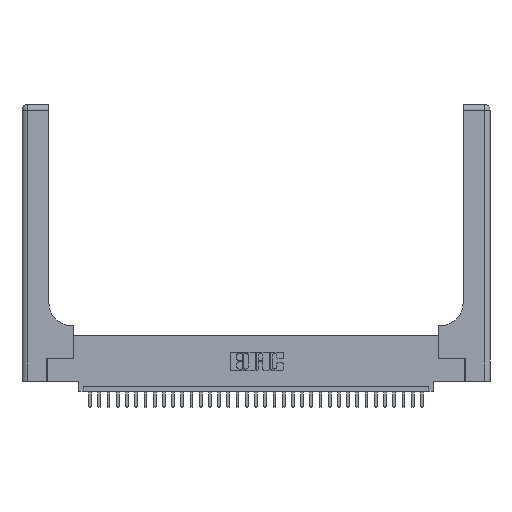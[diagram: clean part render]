
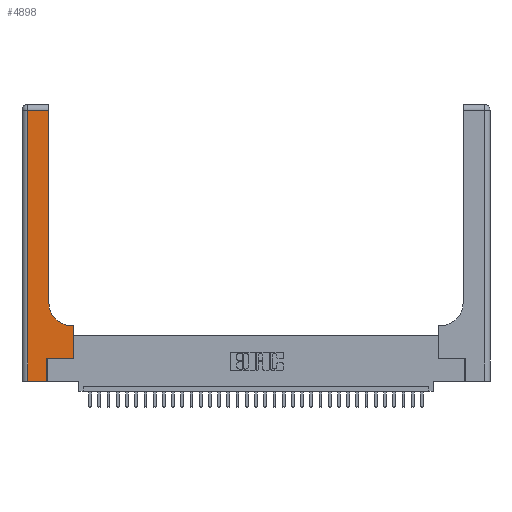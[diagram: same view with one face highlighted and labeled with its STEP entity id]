
A CAD part, top view. The second image highlights one B-rep face of the part: STEP entity #4898.
In plain terms, the highlighted planar face has unit normal (0, 0, 1).
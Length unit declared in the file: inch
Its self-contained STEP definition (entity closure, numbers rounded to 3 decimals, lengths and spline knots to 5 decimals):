
#101 = VERTEX_POINT ( 'NONE', #15010 ) ;
#914 = VERTEX_POINT ( 'NONE', #10750 ) ;
#1410 = CARTESIAN_POINT ( 'NONE',  ( 0.06, 3., 0.37 ) ) ;
#1652 = CARTESIAN_POINT ( 'NONE',  ( 0.5585, 0.6, 0.37 ) ) ;
#3017 = DIRECTION ( 'NONE',  ( 0., 1., 0. ) ) ;
#3112 = EDGE_CURVE ( 'NONE', #20551, #27296, #12421, .T. ) ;
#3585 = CARTESIAN_POINT ( 'NONE',  ( 0., 2.94, 0.37 ) ) ;
#4898 = ADVANCED_FACE ( 'NONE', ( #30278 ), #31726, .F. ) ;
#5495 = DIRECTION ( 'NONE',  ( 0., 0., -1. ) ) ;
#5794 = LINE ( 'NONE', #6633, #22554 ) ;
#5847 = ORIENTED_EDGE ( 'NONE', *, *, #11827, .T. ) ;
#5917 = VERTEX_POINT ( 'NONE', #32059 ) ;
#6014 = CIRCLE ( 'NONE', #30417, 0.25 ) ;
#6218 = DIRECTION ( 'NONE',  ( 0., -1., 0. ) ) ;
#6274 = DIRECTION ( 'NONE',  ( 0., 1., 0. ) ) ;
#6325 = ORIENTED_EDGE ( 'NONE', *, *, #32760, .T. ) ;
#6549 = VECTOR ( 'NONE', #22015, 39.37008 ) ;
#6633 = CARTESIAN_POINT ( 'NONE',  ( 0.5585, 0.25, 0.37 ) ) ;
#7405 = LINE ( 'NONE', #21415, #28686 ) ;
#8240 = CARTESIAN_POINT ( 'NONE',  ( 0., 3., 0.37 ) ) ;
#8337 = LINE ( 'NONE', #1410, #32090 ) ;
#8367 = DIRECTION ( 'NONE',  ( 1., 0., 0. ) ) ;
#8382 = EDGE_CURVE ( 'NONE', #914, #101, #29409, .T. ) ;
#8520 = CARTESIAN_POINT ( 'NONE',  ( 0.269, 0., 0.37 ) ) ;
#8709 = ORIENTED_EDGE ( 'NONE', *, *, #16047, .T. ) ;
#9122 = ORIENTED_EDGE ( 'NONE', *, *, #3112, .T. ) ;
#9137 = VERTEX_POINT ( 'NONE', #15491 ) ;
#9148 = DIRECTION ( 'NONE',  ( 0., 0., -1. ) ) ;
#9297 = ORIENTED_EDGE ( 'NONE', *, *, #15444, .T. ) ;
#9334 = VECTOR ( 'NONE', #6274, 39.37008 ) ;
#9368 = DIRECTION ( 'NONE',  ( 0., 1., 0. ) ) ;
#10034 = AXIS2_PLACEMENT_3D ( 'NONE', #8240, #5495, #16240 ) ;
#10750 = CARTESIAN_POINT ( 'NONE',  ( 0.269, 0.25, 0.37 ) ) ;
#11162 = DIRECTION ( 'NONE',  ( 1., 0., 0. ) ) ;
#11827 = EDGE_CURVE ( 'NONE', #5917, #28578, #15257, .T. ) ;
#12421 = LINE ( 'NONE', #21378, #31283 ) ;
#12800 = CARTESIAN_POINT ( 'NONE',  ( 0.06, 0., 0.37 ) ) ;
#13946 = CARTESIAN_POINT ( 'NONE',  ( 0.2915, 3., 0.37 ) ) ;
#14524 = EDGE_CURVE ( 'NONE', #28578, #20551, #8337, .T. ) ;
#14715 = EDGE_LOOP ( 'NONE', ( #21455, #5847, #18356, #9122, #15242, #21396, #9297, #8709, #6325 ) ) ;
#15010 = CARTESIAN_POINT ( 'NONE',  ( 0.5585, 0.25, 0.37 ) ) ;
#15242 = ORIENTED_EDGE ( 'NONE', *, *, #26597, .T. ) ;
#15257 = LINE ( 'NONE', #3585, #28356 ) ;
#15444 = EDGE_CURVE ( 'NONE', #101, #21053, #5794, .T. ) ;
#15491 = CARTESIAN_POINT ( 'NONE',  ( 0.5415, 0.6, 0.37 ) ) ;
#16047 = EDGE_CURVE ( 'NONE', #21053, #9137, #17986, .T. ) ;
#16240 = DIRECTION ( 'NONE',  ( -1., 0., 0. ) ) ;
#16301 = LINE ( 'NONE', #13946, #9334 ) ;
#17802 = EDGE_CURVE ( 'NONE', #28194, #5917, #16301, .T. ) ;
#17986 = LINE ( 'NONE', #29734, #6549 ) ;
#18356 = ORIENTED_EDGE ( 'NONE', *, *, #14524, .T. ) ;
#20081 = CARTESIAN_POINT ( 'NONE',  ( 0.2915, 0.85, 0.37 ) ) ;
#20551 = VERTEX_POINT ( 'NONE', #12800 ) ;
#21053 = VERTEX_POINT ( 'NONE', #1652 ) ;
#21378 = CARTESIAN_POINT ( 'NONE',  ( 0., 0., 0.37 ) ) ;
#21396 = ORIENTED_EDGE ( 'NONE', *, *, #8382, .T. ) ;
#21415 = CARTESIAN_POINT ( 'NONE',  ( 0.269, 0., 0.37 ) ) ;
#21455 = ORIENTED_EDGE ( 'NONE', *, *, #17802, .T. ) ;
#21792 = CARTESIAN_POINT ( 'NONE',  ( 0.06, 2.94, 0.37 ) ) ;
#22015 = DIRECTION ( 'NONE',  ( -1., 0., 0. ) ) ;
#22554 = VECTOR ( 'NONE', #9368, 39.37008 ) ;
#23676 = VECTOR ( 'NONE', #11162, 39.37008 ) ;
#26597 = EDGE_CURVE ( 'NONE', #27296, #914, #7405, .T. ) ;
#26695 = CARTESIAN_POINT ( 'NONE',  ( 0.269, 0.25, 0.37 ) ) ;
#27296 = VERTEX_POINT ( 'NONE', #8520 ) ;
#27438 = DIRECTION ( 'NONE',  ( 1., 0., 0. ) ) ;
#28194 = VERTEX_POINT ( 'NONE', #20081 ) ;
#28356 = VECTOR ( 'NONE', #29578, 39.37008 ) ;
#28578 = VERTEX_POINT ( 'NONE', #21792 ) ;
#28686 = VECTOR ( 'NONE', #3017, 39.37008 ) ;
#29409 = LINE ( 'NONE', #26695, #23676 ) ;
#29578 = DIRECTION ( 'NONE',  ( -1., 0., 0. ) ) ;
#29734 = CARTESIAN_POINT ( 'NONE',  ( 0.2915, 0.6, 0.37 ) ) ;
#30278 = FACE_OUTER_BOUND ( 'NONE', #14715, .T. ) ;
#30417 = AXIS2_PLACEMENT_3D ( 'NONE', #32506, #9148, #27438 ) ;
#31283 = VECTOR ( 'NONE', #8367, 39.37008 ) ;
#31726 = PLANE ( 'NONE',  #10034 ) ;
#32059 = CARTESIAN_POINT ( 'NONE',  ( 0.2915, 2.94, 0.37 ) ) ;
#32090 = VECTOR ( 'NONE', #6218, 39.37008 ) ;
#32506 = CARTESIAN_POINT ( 'NONE',  ( 0.5415, 0.85, 0.37 ) ) ;
#32760 = EDGE_CURVE ( 'NONE', #9137, #28194, #6014, .T. ) ;
